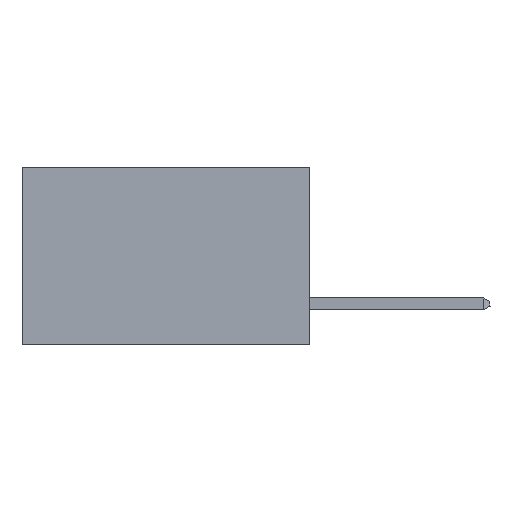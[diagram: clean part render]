
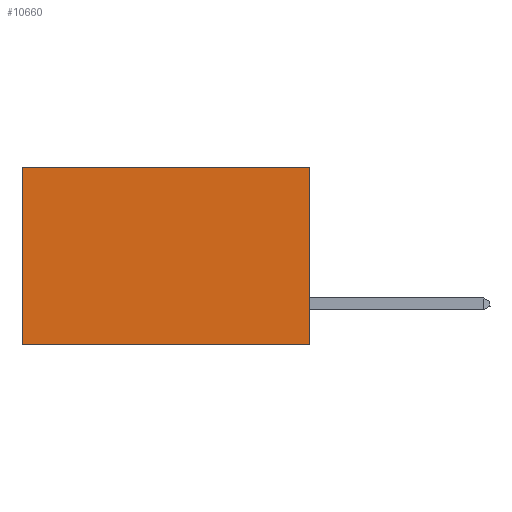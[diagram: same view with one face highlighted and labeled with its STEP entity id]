
A CAD part, left-side view. The second image highlights one B-rep face of the part: STEP entity #10660.
In plain terms, the highlighted planar face has unit normal (-1, 0, 0).
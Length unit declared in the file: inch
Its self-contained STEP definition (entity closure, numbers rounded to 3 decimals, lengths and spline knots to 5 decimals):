
#550 = CARTESIAN_POINT ( 'NONE',  ( 0.2875, 0., 0. ) ) ;
#1720 = AXIS2_PLACEMENT_3D ( 'NONE', #16730, #16867, #37942 ) ;
#2721 = EDGE_CURVE ( 'NONE', #21027, #6330, #13724, .T. ) ;
#4088 = CARTESIAN_POINT ( 'NONE',  ( 0.2875, 0., 0. ) ) ;
#4331 = CARTESIAN_POINT ( 'NONE',  ( 0.2875, 0., 0. ) ) ;
#4777 = VECTOR ( 'NONE', #30744, 39.37008 ) ;
#6330 = VERTEX_POINT ( 'NONE', #28270 ) ;
#10660 = ADVANCED_FACE ( 'NONE', ( #21801 ), #25991, .F. ) ;
#11753 = LINE ( 'NONE', #4331, #24039 ) ;
#11809 = EDGE_CURVE ( 'NONE', #15864, #12752, #11753, .T. ) ;
#12752 = VERTEX_POINT ( 'NONE', #27631 ) ;
#13724 = LINE ( 'NONE', #29942, #30169 ) ;
#15817 = ORIENTED_EDGE ( 'NONE', *, *, #33914, .T. ) ;
#15864 = VERTEX_POINT ( 'NONE', #4088 ) ;
#16730 = CARTESIAN_POINT ( 'NONE',  ( 0.2875, 0., 0. ) ) ;
#16772 = CARTESIAN_POINT ( 'NONE',  ( 0.2875, 0., -0.37 ) ) ;
#16808 = DIRECTION ( 'NONE',  ( 0., 0., -1. ) ) ;
#16867 = DIRECTION ( 'NONE',  ( 1., 0., 0. ) ) ;
#19973 = CARTESIAN_POINT ( 'NONE',  ( 0.2875, 0.6, 0. ) ) ;
#20942 = ORIENTED_EDGE ( 'NONE', *, *, #21960, .F. ) ;
#21027 = VERTEX_POINT ( 'NONE', #19973 ) ;
#21801 = FACE_OUTER_BOUND ( 'NONE', #29875, .T. ) ;
#21960 = EDGE_CURVE ( 'NONE', #12752, #6330, #23974, .T. ) ;
#22129 = LINE ( 'NONE', #550, #4777 ) ;
#23974 = LINE ( 'NONE', #16772, #30935 ) ;
#24039 = VECTOR ( 'NONE', #16808, 39.37008 ) ;
#25991 = PLANE ( 'NONE',  #1720 ) ;
#26333 = ORIENTED_EDGE ( 'NONE', *, *, #11809, .F. ) ;
#27631 = CARTESIAN_POINT ( 'NONE',  ( 0.2875, 0., -0.37 ) ) ;
#28270 = CARTESIAN_POINT ( 'NONE',  ( 0.2875, 0.6, -0.37 ) ) ;
#29569 = DIRECTION ( 'NONE',  ( 0., 0., -1. ) ) ;
#29875 = EDGE_LOOP ( 'NONE', ( #33721, #20942, #26333, #15817 ) ) ;
#29942 = CARTESIAN_POINT ( 'NONE',  ( 0.2875, 0.6, 0. ) ) ;
#30169 = VECTOR ( 'NONE', #29569, 39.37008 ) ;
#30744 = DIRECTION ( 'NONE',  ( 0., 1., 0. ) ) ;
#30935 = VECTOR ( 'NONE', #37715, 39.37008 ) ;
#33721 = ORIENTED_EDGE ( 'NONE', *, *, #2721, .T. ) ;
#33914 = EDGE_CURVE ( 'NONE', #15864, #21027, #22129, .T. ) ;
#37715 = DIRECTION ( 'NONE',  ( 0., 1., 0. ) ) ;
#37942 = DIRECTION ( 'NONE',  ( 0., 0., -1. ) ) ;
